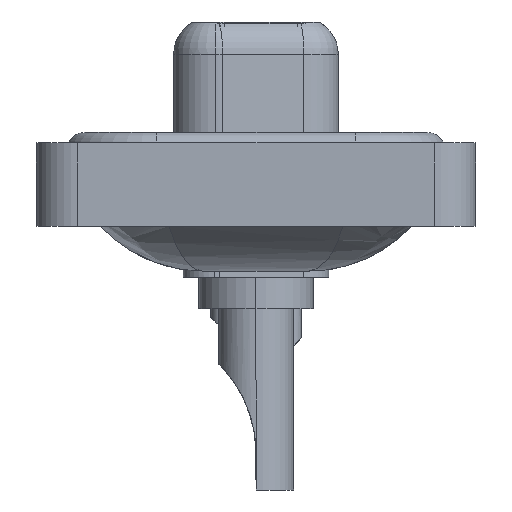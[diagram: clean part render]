
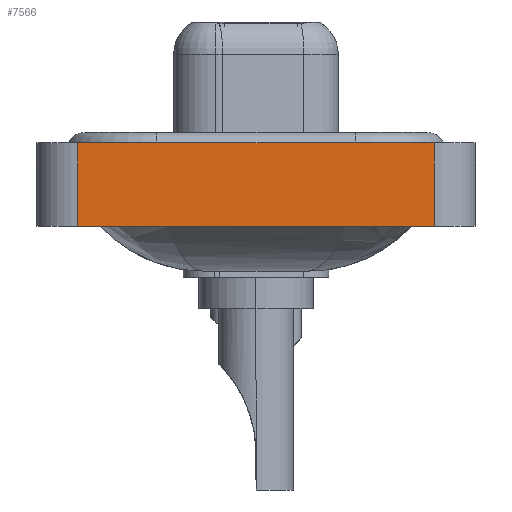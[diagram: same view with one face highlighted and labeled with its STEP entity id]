
A CAD part, left-side view. The second image highlights one B-rep face of the part: STEP entity #7566.
In plain terms, the highlighted planar face has unit normal (-1, 0, 0).
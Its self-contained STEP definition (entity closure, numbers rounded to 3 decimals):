
#381 = EDGE_CURVE ( 'NONE', #13527, #19385, #11580, .T. ) ;
#996 = ORIENTED_EDGE ( 'NONE', *, *, #4365, .F. ) ;
#4365 = EDGE_CURVE ( 'NONE', #13527, #22294, #18436, .T. ) ;
#5910 = VECTOR ( 'NONE', #10574, 1000. ) ;
#6794 = EDGE_CURVE ( 'NONE', #19385, #10464, #17396, .T. ) ;
#6992 = EDGE_CURVE ( 'NONE', #22294, #10464, #8886, .T. ) ;
#7201 = FACE_OUTER_BOUND ( 'NONE', #10380, .T. ) ;
#7566 = ADVANCED_FACE ( 'NONE', ( #7201 ), #22793, .T. ) ;
#8038 = CARTESIAN_POINT ( 'NONE',  ( -7.35, -8.55, -3.6 ) ) ;
#8228 = ORIENTED_EDGE ( 'NONE', *, *, #381, .T. ) ;
#8886 = LINE ( 'NONE', #16477, #24308 ) ;
#9337 = DIRECTION ( 'NONE',  ( 0., -1., 0. ) ) ;
#9398 = CARTESIAN_POINT ( 'NONE',  ( -7.35, -8.55, -3.6 ) ) ;
#10380 = EDGE_LOOP ( 'NONE', ( #17270, #22646, #996, #8228 ) ) ;
#10464 = VERTEX_POINT ( 'NONE', #11403 ) ;
#10574 = DIRECTION ( 'NONE',  ( 0., 0., 1. ) ) ;
#11403 = CARTESIAN_POINT ( 'NONE',  ( -7.35, -8.55, 0.4 ) ) ;
#11580 = LINE ( 'NONE', #16939, #18179 ) ;
#11975 = VECTOR ( 'NONE', #15260, 1000. ) ;
#12695 = DIRECTION ( 'NONE',  ( 0., 0., 1. ) ) ;
#13527 = VERTEX_POINT ( 'NONE', #16102 ) ;
#14685 = CARTESIAN_POINT ( 'NONE',  ( -7.35, -8.55, -3.6 ) ) ;
#15260 = DIRECTION ( 'NONE',  ( 0., 0., 1. ) ) ;
#16102 = CARTESIAN_POINT ( 'NONE',  ( -7.35, 8.55, -3.6 ) ) ;
#16477 = CARTESIAN_POINT ( 'NONE',  ( -7.35, -8.55, 0.4 ) ) ;
#16937 = DIRECTION ( 'NONE',  ( -1., 0., 0. ) ) ;
#16939 = CARTESIAN_POINT ( 'NONE',  ( -7.35, -8.55, -3.6 ) ) ;
#17270 = ORIENTED_EDGE ( 'NONE', *, *, #6794, .T. ) ;
#17396 = LINE ( 'NONE', #8038, #11975 ) ;
#18179 = VECTOR ( 'NONE', #9337, 1000. ) ;
#18253 = DIRECTION ( 'NONE',  ( 0., -1., 0. ) ) ;
#18436 = LINE ( 'NONE', #20571, #5910 ) ;
#19385 = VERTEX_POINT ( 'NONE', #9398 ) ;
#20571 = CARTESIAN_POINT ( 'NONE',  ( -7.35, 8.55, -3.6 ) ) ;
#22294 = VERTEX_POINT ( 'NONE', #23500 ) ;
#22646 = ORIENTED_EDGE ( 'NONE', *, *, #6992, .F. ) ;
#22793 = PLANE ( 'NONE',  #23782 ) ;
#23500 = CARTESIAN_POINT ( 'NONE',  ( -7.35, 8.55, 0.4 ) ) ;
#23782 = AXIS2_PLACEMENT_3D ( 'NONE', #14685, #16937, #12695 ) ;
#24308 = VECTOR ( 'NONE', #18253, 1000. ) ;
